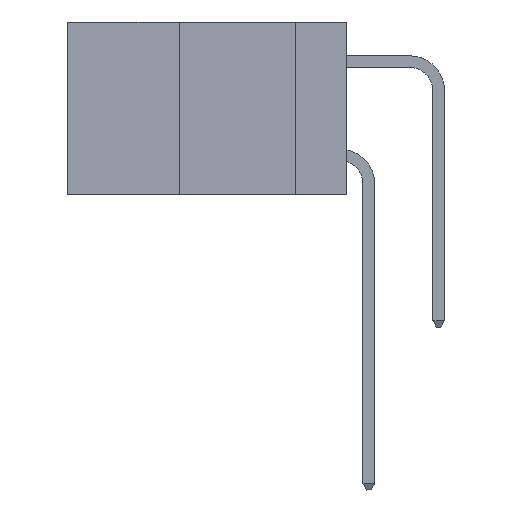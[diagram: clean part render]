
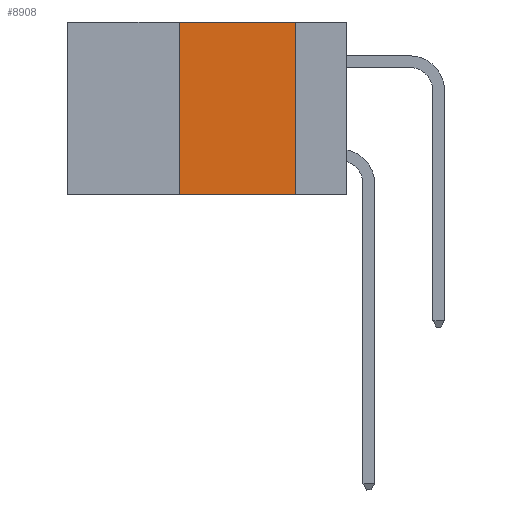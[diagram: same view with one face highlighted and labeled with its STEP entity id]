
A CAD part, left-side view. The second image highlights one B-rep face of the part: STEP entity #8908.
In plain terms, the highlighted planar face has unit normal (-1, 0, 0).
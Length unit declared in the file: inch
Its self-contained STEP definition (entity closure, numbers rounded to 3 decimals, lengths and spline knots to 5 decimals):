
#1833 = CARTESIAN_POINT ( 'NONE',  ( 0., 0.11, -0.37 ) ) ;
#1912 = CARTESIAN_POINT ( 'NONE',  ( 0., 0.11, 0. ) ) ;
#2398 = DIRECTION ( 'NONE',  ( 0., -1., 0. ) ) ;
#3849 = VERTEX_POINT ( 'NONE', #16673 ) ;
#4404 = EDGE_CURVE ( 'NONE', #12704, #15352, #14316, .T. ) ;
#4447 = CARTESIAN_POINT ( 'NONE',  ( 0., 0.6, 0. ) ) ;
#4635 = DIRECTION ( 'NONE',  ( 1., 0., 0. ) ) ;
#4703 = EDGE_CURVE ( 'NONE', #12704, #15317, #10159, .T. ) ;
#4735 = LINE ( 'NONE', #1912, #10113 ) ;
#4819 = VECTOR ( 'NONE', #15146, 39.37008 ) ;
#5113 = CARTESIAN_POINT ( 'NONE',  ( 0., 0.36, -0.37 ) ) ;
#5833 = EDGE_CURVE ( 'NONE', #3849, #15352, #4735, .T. ) ;
#6648 = VECTOR ( 'NONE', #15318, 39.37008 ) ;
#6837 = ORIENTED_EDGE ( 'NONE', *, *, #9865, .F. ) ;
#8721 = CARTESIAN_POINT ( 'NONE',  ( 0., 0.36, 0. ) ) ;
#8778 = FACE_OUTER_BOUND ( 'NONE', #17168, .T. ) ;
#8908 = ADVANCED_FACE ( 'NONE', ( #8778 ), #12544, .F. ) ;
#9865 = EDGE_CURVE ( 'NONE', #15317, #3849, #10826, .T. ) ;
#10113 = VECTOR ( 'NONE', #11185, 39.37008 ) ;
#10159 = LINE ( 'NONE', #8721, #6648 ) ;
#10784 = VECTOR ( 'NONE', #2398, 39.37008 ) ;
#10826 = LINE ( 'NONE', #4447, #4819 ) ;
#11085 = ORIENTED_EDGE ( 'NONE', *, *, #4703, .F. ) ;
#11185 = DIRECTION ( 'NONE',  ( 0., 0., -1. ) ) ;
#12544 = PLANE ( 'NONE',  #13715 ) ;
#12704 = VERTEX_POINT ( 'NONE', #5113 ) ;
#13715 = AXIS2_PLACEMENT_3D ( 'NONE', #13819, #4635, #15175 ) ;
#13819 = CARTESIAN_POINT ( 'NONE',  ( 0., 0.6, 0. ) ) ;
#14027 = ORIENTED_EDGE ( 'NONE', *, *, #4404, .T. ) ;
#14316 = LINE ( 'NONE', #16943, #10784 ) ;
#14952 = ORIENTED_EDGE ( 'NONE', *, *, #5833, .F. ) ;
#15146 = DIRECTION ( 'NONE',  ( 0., -1., 0. ) ) ;
#15175 = DIRECTION ( 'NONE',  ( 0., 0., -1. ) ) ;
#15317 = VERTEX_POINT ( 'NONE', #16336 ) ;
#15318 = DIRECTION ( 'NONE',  ( 0., 0., 1. ) ) ;
#15352 = VERTEX_POINT ( 'NONE', #1833 ) ;
#16336 = CARTESIAN_POINT ( 'NONE',  ( 0., 0.36, 0. ) ) ;
#16673 = CARTESIAN_POINT ( 'NONE',  ( 0., 0.11, 0. ) ) ;
#16943 = CARTESIAN_POINT ( 'NONE',  ( 0., 0.6, -0.37 ) ) ;
#17168 = EDGE_LOOP ( 'NONE', ( #14952, #6837, #11085, #14027 ) ) ;
